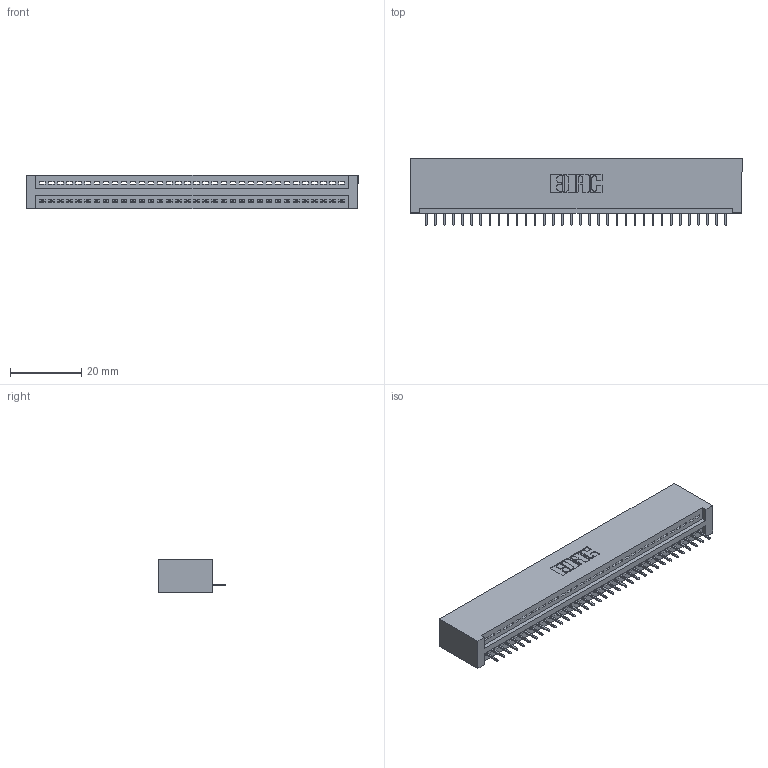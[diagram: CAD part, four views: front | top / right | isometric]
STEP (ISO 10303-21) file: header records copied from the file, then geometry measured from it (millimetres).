
FILE_DESCRIPTION (( 'STEP AP203' ), '1' );
FILE_NAME ('395-034-525-101.STEP', '2020-09-23T22:00:17', ( '' ), ( '' ), 'SwSTEP 2.0', 'SolidWorks 2020', '' );
FILE_SCHEMA (( 'CONFIG_CONTROL_DESIGN' ));
Length unit declared in the file: inch
Products named in the file (3): 345 Part_No Mounting Lugs; 395-034-525-101; 345-292-001_345-293-125
Assembly tree (35 placements, depth 2):
  395-034-525-101
    345 Part_No Mounting Lugs
    345-292-001_345-293-125  x34
Bounding box: 92.96 x 18.72 x 9.4 mm (x, y, z)
Volume: 9209.8 mm3; surface area: 11857.5 mm2
Topology: 35 solids, 35 shells, 2226 faces, 6437 edges, 4154 vertices
Faces by surface type: plane 1640, cylinder 586
Entity records: 26463 total; most frequent: CARTESIAN_POINT 4590, ORIENTED_EDGE 4558, DIRECTION 4015, EDGE_CURVE 2279, LINE 2023, VECTOR 2023, VERTEX_POINT 1514, AXIS2_PLACEMENT_3D 996
